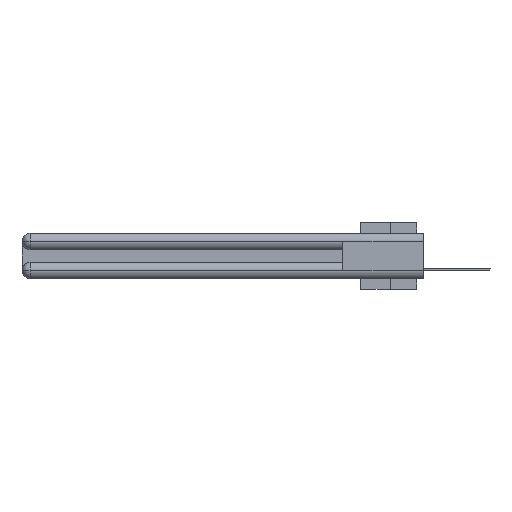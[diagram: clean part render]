
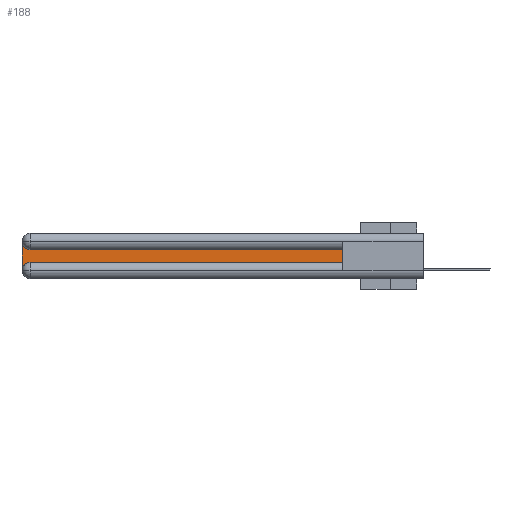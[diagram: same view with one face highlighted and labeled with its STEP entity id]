
A CAD part, left-side view. The second image highlights one B-rep face of the part: STEP entity #188.
In plain terms, the highlighted planar face has unit normal (-1, 0, 0).
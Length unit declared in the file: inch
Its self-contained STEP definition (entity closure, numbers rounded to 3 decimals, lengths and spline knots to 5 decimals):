
#188 = ADVANCED_FACE ( 'NONE', ( #5764 ), #8204, .F. ) ;
#347 = VERTEX_POINT ( 'NONE', #20963 ) ;
#595 = VERTEX_POINT ( 'NONE', #28462 ) ;
#677 = VECTOR ( 'NONE', #11920, 39.37008 ) ;
#1018 = CIRCLE ( 'NONE', #22031, 0.06 ) ;
#1500 = VECTOR ( 'NONE', #13754, 39.37008 ) ;
#2272 = LINE ( 'NONE', #36852, #1500 ) ;
#3462 = LINE ( 'NONE', #14945, #27475 ) ;
#3492 = DIRECTION ( 'NONE',  ( 1., 0., 0. ) ) ;
#3692 = AXIS2_PLACEMENT_3D ( 'NONE', #22843, #11768, #8938 ) ;
#3919 = VECTOR ( 'NONE', #33666, 39.37008 ) ;
#4074 = CARTESIAN_POINT ( 'NONE',  ( 0.075, 3., -0.2775 ) ) ;
#5082 = EDGE_CURVE ( 'NONE', #31957, #347, #9271, .T. ) ;
#5764 = FACE_OUTER_BOUND ( 'NONE', #19196, .T. ) ;
#5921 = CARTESIAN_POINT ( 'NONE',  ( 0.075, 3., -0.0625 ) ) ;
#6135 = DIRECTION ( 'NONE',  ( 0., 0., -1. ) ) ;
#6444 = CARTESIAN_POINT ( 'NONE',  ( 0.075, 0.6, -0.2175 ) ) ;
#8091 = CARTESIAN_POINT ( 'NONE',  ( 0.075, 0.6, -0.2175 ) ) ;
#8204 = PLANE ( 'NONE',  #17678 ) ;
#8938 = DIRECTION ( 'NONE',  ( 0., 0., -1. ) ) ;
#9150 = CARTESIAN_POINT ( 'NONE',  ( 0.075, 2.94, -0.0625 ) ) ;
#9271 = LINE ( 'NONE', #6444, #677 ) ;
#9952 = EDGE_CURVE ( 'NONE', #595, #24246, #2272, .T. ) ;
#10740 = VERTEX_POINT ( 'NONE', #4074 ) ;
#11303 = LINE ( 'NONE', #8091, #3919 ) ;
#11768 = DIRECTION ( 'NONE',  ( 1., 0., 0. ) ) ;
#11920 = DIRECTION ( 'NONE',  ( 0., -1., 0. ) ) ;
#12488 = ORIENTED_EDGE ( 'NONE', *, *, #9952, .T. ) ;
#12999 = CARTESIAN_POINT ( 'NONE',  ( 0.075, 2.94, -0.2175 ) ) ;
#13754 = DIRECTION ( 'NONE',  ( 0., 1., 0. ) ) ;
#14194 = ORIENTED_EDGE ( 'NONE', *, *, #5082, .T. ) ;
#14304 = EDGE_CURVE ( 'NONE', #23774, #10740, #3462, .T. ) ;
#14945 = CARTESIAN_POINT ( 'NONE',  ( 0.075, 3., -0.2175 ) ) ;
#15810 = EDGE_CURVE ( 'NONE', #24246, #23774, #1018, .T. ) ;
#16267 = CIRCLE ( 'NONE', #3692, 0.06 ) ;
#17054 = CARTESIAN_POINT ( 'NONE',  ( 0.075, 3., -0.1225 ) ) ;
#17678 = AXIS2_PLACEMENT_3D ( 'NONE', #17054, #30956, #28324 ) ;
#17941 = DIRECTION ( 'NONE',  ( 0., 0., -1. ) ) ;
#18370 = ORIENTED_EDGE ( 'NONE', *, *, #14304, .T. ) ;
#19196 = EDGE_LOOP ( 'NONE', ( #12488, #22591, #18370, #25108, #14194, #22072 ) ) ;
#20963 = CARTESIAN_POINT ( 'NONE',  ( 0.075, 0.6, -0.2175 ) ) ;
#21449 = EDGE_CURVE ( 'NONE', #10740, #31957, #16267, .T. ) ;
#22031 = AXIS2_PLACEMENT_3D ( 'NONE', #9150, #3492, #6135 ) ;
#22072 = ORIENTED_EDGE ( 'NONE', *, *, #29087, .T. ) ;
#22591 = ORIENTED_EDGE ( 'NONE', *, *, #15810, .T. ) ;
#22843 = CARTESIAN_POINT ( 'NONE',  ( 0.075, 2.94, -0.2775 ) ) ;
#23774 = VERTEX_POINT ( 'NONE', #5921 ) ;
#24035 = CARTESIAN_POINT ( 'NONE',  ( 0.075, 2.94, -0.1225 ) ) ;
#24246 = VERTEX_POINT ( 'NONE', #24035 ) ;
#25108 = ORIENTED_EDGE ( 'NONE', *, *, #21449, .T. ) ;
#27475 = VECTOR ( 'NONE', #17941, 39.37008 ) ;
#28324 = DIRECTION ( 'NONE',  ( 0., 0., -1. ) ) ;
#28462 = CARTESIAN_POINT ( 'NONE',  ( 0.075, 0.6, -0.1225 ) ) ;
#29087 = EDGE_CURVE ( 'NONE', #347, #595, #11303, .T. ) ;
#30956 = DIRECTION ( 'NONE',  ( 1., 0., 0. ) ) ;
#31957 = VERTEX_POINT ( 'NONE', #12999 ) ;
#33666 = DIRECTION ( 'NONE',  ( 0., 0., 1. ) ) ;
#36852 = CARTESIAN_POINT ( 'NONE',  ( 0.075, 0.6, -0.1225 ) ) ;
